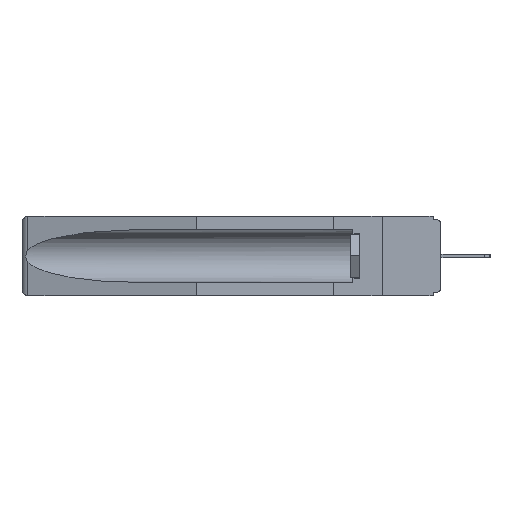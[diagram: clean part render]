
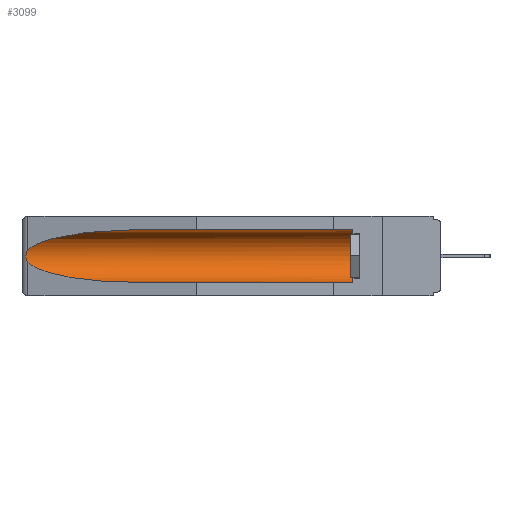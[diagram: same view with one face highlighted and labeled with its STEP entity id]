
A CAD part, left-side view. The second image highlights one B-rep face of the part: STEP entity #3099.
In plain terms, the highlighted cylindrical face has radius 2.857 mm (diameter 5.715 mm), a partial arc.
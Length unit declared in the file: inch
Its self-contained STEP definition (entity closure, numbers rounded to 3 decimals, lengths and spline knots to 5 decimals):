
#932 = CARTESIAN_POINT ( 'NONE',  ( 0.155, 1.07973, -0.059 ) ) ;
#940 = B_SPLINE_CURVE_WITH_KNOTS ( 'NONE', 3,
 ( #19423, #3572, #7564, #15687, #23310, #17625, #7951, #25380, #23181, #9484 ),
 .UNSPECIFIED., .F., .F.,
 ( 4, 2, 2, 2, 4 ),
 ( 0., 0.00029, 0.00058, 0.00087, 0.00117 ),
 .UNSPECIFIED. ) ;
#1479 = EDGE_CURVE ( 'NONE', #20110, #6561, #20079, .T. ) ;
#1814 = DIRECTION ( 'NONE',  ( 0., 1., 0. ) ) ;
#1863 = EDGE_CURVE ( 'NONE', #20531, #6287, #5020, .T. ) ;
#2372 = CARTESIAN_POINT ( 'NONE',  ( 0.155, 1.07973, -0.284 ) ) ;
#2408 = CARTESIAN_POINT ( 'NONE',  ( 0.155, -0.30754, -0.059 ) ) ;
#2592 = CARTESIAN_POINT ( 'NONE',  ( 0.26537, 1.52718, -0.14972 ) ) ;
#3099 = ADVANCED_FACE ( 'NONE', ( #23226 ), #5553, .F. ) ;
#3175 = ORIENTED_EDGE ( 'NONE', *, *, #12408, .T. ) ;
#3572 = CARTESIAN_POINT ( 'NONE',  ( 0.26597, 1.52961, -0.15275 ) ) ;
#4008 = CARTESIAN_POINT ( 'NONE',  ( 0.155, 0.126, -0.284 ) ) ;
#5020 =( BOUNDED_CURVE ( )  B_SPLINE_CURVE ( 3, ( #12209, #20045, #17729, #2372 ),
 .UNSPECIFIED., .F., .F. ) 
 B_SPLINE_CURVE_WITH_KNOTS ( ( 4, 4 ),
 ( 0.1948, 1.5708 ),
 .UNSPECIFIED. ) 
 CURVE ( )  GEOMETRIC_REPRESENTATION_ITEM ( )  RATIONAL_B_SPLINE_CURVE ( ( 1., 0.848, 0.848, 1. ) ) 
 REPRESENTATION_ITEM ( '' )  );
#5450 = VECTOR ( 'NONE', #17081, 39.37008 ) ;
#5553 = CYLINDRICAL_SURFACE ( 'NONE', #21886, 0.1125 ) ;
#5815 = ORIENTED_EDGE ( 'NONE', *, *, #1479, .T. ) ;
#6259 = AXIS2_PLACEMENT_3D ( 'NONE', #9119, #18676, #20601 ) ;
#6287 = VERTEX_POINT ( 'NONE', #13211 ) ;
#6561 = VERTEX_POINT ( 'NONE', #932 ) ;
#7108 = VERTEX_POINT ( 'NONE', #2592 ) ;
#7564 = CARTESIAN_POINT ( 'NONE',  ( 0.26654, 1.53092, -0.15636 ) ) ;
#7951 = CARTESIAN_POINT ( 'NONE',  ( 0.2673, 1.53269, -0.17917 ) ) ;
#8806 = CARTESIAN_POINT ( 'NONE',  ( 0.155, 1.07973, -0.059 ) ) ;
#8892 = CARTESIAN_POINT ( 'NONE',  ( 0.155, 0.126, -0.059 ) ) ;
#9118 = VERTEX_POINT ( 'NONE', #4008 ) ;
#9119 = CARTESIAN_POINT ( 'NONE',  ( 0.155, 0.126, -0.1715 ) ) ;
#9290 = CARTESIAN_POINT ( 'NONE',  ( 0.155, -0.30754, -0.1715 ) ) ;
#9484 = CARTESIAN_POINT ( 'NONE',  ( 0.26537, 1.52718, -0.19328 ) ) ;
#9668 = DIRECTION ( 'NONE',  ( 0., 0., 1. ) ) ;
#10057 = ORIENTED_EDGE ( 'NONE', *, *, #11122, .T. ) ;
#10736 = CARTESIAN_POINT ( 'NONE',  ( 0.26537, 1.52718, -0.14972 ) ) ;
#11122 = EDGE_CURVE ( 'NONE', #6561, #7108, #19857, .T. ) ;
#12209 = CARTESIAN_POINT ( 'NONE',  ( 0.26537, 1.52718, -0.19328 ) ) ;
#12357 = VECTOR ( 'NONE', #20207, 39.37008 ) ;
#12408 = EDGE_CURVE ( 'NONE', #7108, #20531, #940, .T. ) ;
#12641 = CARTESIAN_POINT ( 'NONE',  ( 0.26537, 1.52718, -0.19328 ) ) ;
#13211 = CARTESIAN_POINT ( 'NONE',  ( 0.155, 1.07973, -0.284 ) ) ;
#15085 = ORIENTED_EDGE ( 'NONE', *, *, #1863, .T. ) ;
#15687 = CARTESIAN_POINT ( 'NONE',  ( 0.2673, 1.5327, -0.16383 ) ) ;
#17081 = DIRECTION ( 'NONE',  ( 0., 1., 0. ) ) ;
#17625 = CARTESIAN_POINT ( 'NONE',  ( 0.2675, 1.53308, -0.17534 ) ) ;
#17729 = CARTESIAN_POINT ( 'NONE',  ( 0.21114, 1.30732, -0.284 ) ) ;
#18676 = DIRECTION ( 'NONE',  ( 0., -1., 0. ) ) ;
#18736 = CARTESIAN_POINT ( 'NONE',  ( 0.25451, 1.48313, -0.09465 ) ) ;
#19423 = CARTESIAN_POINT ( 'NONE',  ( 0.26537, 1.52718, -0.14972 ) ) ;
#19857 =( BOUNDED_CURVE ( )  B_SPLINE_CURVE ( 3, ( #8806, #20915, #18736, #10736 ),
 .UNSPECIFIED., .F., .F. ) 
 B_SPLINE_CURVE_WITH_KNOTS ( ( 4, 4 ),
 ( 4.71239, 6.08839 ),
 .UNSPECIFIED. ) 
 CURVE ( )  GEOMETRIC_REPRESENTATION_ITEM ( )  RATIONAL_B_SPLINE_CURVE ( ( 1., 0.848, 0.848, 1. ) ) 
 REPRESENTATION_ITEM ( '' )  );
#20045 = CARTESIAN_POINT ( 'NONE',  ( 0.25451, 1.48313, -0.24835 ) ) ;
#20079 = LINE ( 'NONE', #2408, #12357 ) ;
#20110 = VERTEX_POINT ( 'NONE', #8892 ) ;
#20207 = DIRECTION ( 'NONE',  ( 0., 1., 0. ) ) ;
#20520 = EDGE_CURVE ( 'NONE', #9118, #20110, #21075, .T. ) ;
#20531 = VERTEX_POINT ( 'NONE', #12641 ) ;
#20601 = DIRECTION ( 'NONE',  ( 0., 0., 1. ) ) ;
#20697 = CARTESIAN_POINT ( 'NONE',  ( 0.155, -0.30754, -0.284 ) ) ;
#20728 = ORIENTED_EDGE ( 'NONE', *, *, #21009, .F. ) ;
#20915 = CARTESIAN_POINT ( 'NONE',  ( 0.21114, 1.30732, -0.059 ) ) ;
#21009 = EDGE_CURVE ( 'NONE', #9118, #6287, #22629, .T. ) ;
#21075 = CIRCLE ( 'NONE', #6259, 0.1125 ) ;
#21886 = AXIS2_PLACEMENT_3D ( 'NONE', #9290, #1814, #9668 ) ;
#22497 = EDGE_LOOP ( 'NONE', ( #10057, #3175, #15085, #20728, #24997, #5815 ) ) ;
#22629 = LINE ( 'NONE', #20697, #5450 ) ;
#23181 = CARTESIAN_POINT ( 'NONE',  ( 0.26597, 1.5296, -0.19026 ) ) ;
#23226 = FACE_OUTER_BOUND ( 'NONE', #22497, .T. ) ;
#23310 = CARTESIAN_POINT ( 'NONE',  ( 0.2675, 1.53308, -0.16763 ) ) ;
#24997 = ORIENTED_EDGE ( 'NONE', *, *, #20520, .T. ) ;
#25380 = CARTESIAN_POINT ( 'NONE',  ( 0.26655, 1.53094, -0.18657 ) ) ;
